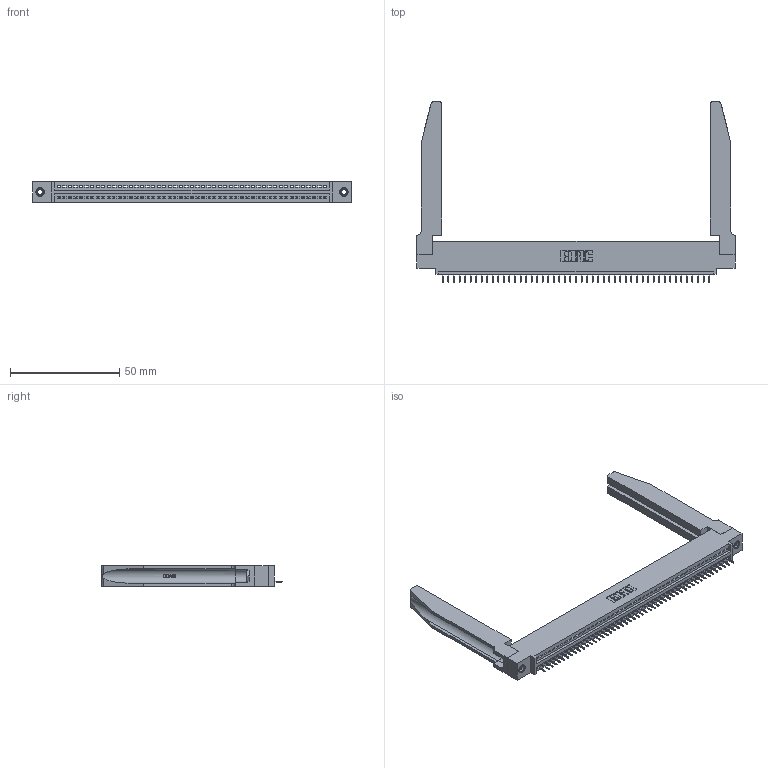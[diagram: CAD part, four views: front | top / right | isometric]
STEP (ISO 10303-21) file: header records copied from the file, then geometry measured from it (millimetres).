
FILE_DESCRIPTION (( 'STEP AP203' ), '1' );
FILE_NAME ('395-049-525-478.STEP', '2020-09-24T09:13:10', ( '' ), ( '' ), 'SwSTEP 2.0', 'SolidWorks 2020', '' );
FILE_SCHEMA (( 'CONFIG_CONTROL_DESIGN' ));
Length unit declared in the file: inch
Products named in the file (5): 345-220-078_345-220-078; 345-292-001_345-293-125; 395-049-525-478; 345-250-001_345-250-001-102; 345 Part_0.110 Offset - 0.156 Dia-TH
Assembly tree (54 placements, depth 2):
  395-049-525-478
    345 Part_0.110 Offset - 0.156 Dia-TH
    345-292-001_345-293-125  x49
    345-250-001_345-250-001-102  x2
    345-220-078_345-220-078  x2
Bounding box: 145.69 x 82.47 x 9.4 mm (x, y, z)
Volume: 21392.6 mm3; surface area: 24458 mm2
Topology: 54 solids, 54 shells, 3402 faces, 9781 edges, 6314 vertices
Faces by surface type: plane 2480, cylinder 870, bspline 36, cone 12, torus 4
Entity records: 40882 total; most frequent: CARTESIAN_POINT 7978, ORIENTED_EDGE 6858, DIRECTION 5965, EDGE_CURVE 3429, LINE 3011, VECTOR 3011, VERTEX_POINT 2276, AXIS2_PLACEMENT_3D 1477
